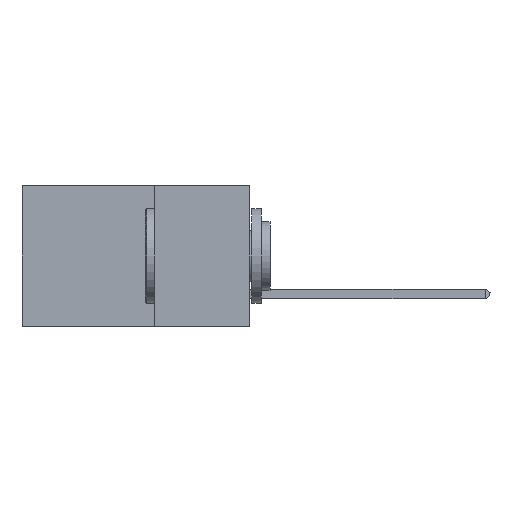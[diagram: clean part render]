
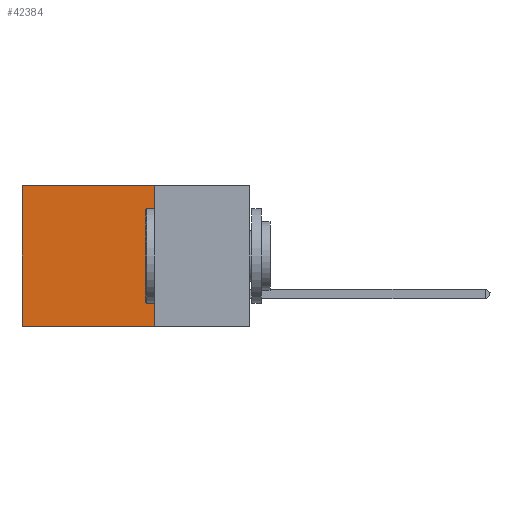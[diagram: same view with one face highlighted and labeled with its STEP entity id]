
A CAD part, left-side view. The second image highlights one B-rep face of the part: STEP entity #42384.
In plain terms, the highlighted planar face has unit normal (-1, 0, 0).
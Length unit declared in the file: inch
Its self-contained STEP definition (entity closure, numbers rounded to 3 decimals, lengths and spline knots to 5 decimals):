
#174 = EDGE_CURVE ( 'NONE', #48204, #36725, #38266, .T. ) ;
#1649 = PLANE ( 'NONE',  #5915 ) ;
#3595 = VERTEX_POINT ( 'NONE', #5203 ) ;
#3979 = VECTOR ( 'NONE', #16102, 39.37008 ) ;
#5203 = CARTESIAN_POINT ( 'NONE',  ( 0.2875, 0.25, -0.37 ) ) ;
#5599 = CARTESIAN_POINT ( 'NONE',  ( 0.2875, 0.25, 0. ) ) ;
#5915 = AXIS2_PLACEMENT_3D ( 'NONE', #5599, #47746, #28613 ) ;
#6799 = CARTESIAN_POINT ( 'NONE',  ( 0.2875, 0.25, -0.37 ) ) ;
#8748 = DIRECTION ( 'NONE',  ( 0., 1., 0. ) ) ;
#12864 = CARTESIAN_POINT ( 'NONE',  ( 0.2875, 0.6, 0. ) ) ;
#14858 = VERTEX_POINT ( 'NONE', #45023 ) ;
#14999 = ORIENTED_EDGE ( 'NONE', *, *, #17855, .F. ) ;
#16102 = DIRECTION ( 'NONE',  ( 0., 0., -1. ) ) ;
#17855 = EDGE_CURVE ( 'NONE', #48204, #3595, #39730, .T. ) ;
#18066 = VECTOR ( 'NONE', #48326, 39.37008 ) ;
#19684 = ORIENTED_EDGE ( 'NONE', *, *, #37822, .T. ) ;
#22387 = CARTESIAN_POINT ( 'NONE',  ( 0.2875, 0.6, 0. ) ) ;
#25393 = VECTOR ( 'NONE', #8748, 39.37008 ) ;
#27623 = CARTESIAN_POINT ( 'NONE',  ( 0.2875, 0.25, 0. ) ) ;
#28146 = ORIENTED_EDGE ( 'NONE', *, *, #39685, .F. ) ;
#28613 = DIRECTION ( 'NONE',  ( 0., 0., -1. ) ) ;
#32929 = FACE_OUTER_BOUND ( 'NONE', #34777, .T. ) ;
#34777 = EDGE_LOOP ( 'NONE', ( #19684, #28146, #14999, #37295 ) ) ;
#36725 = VERTEX_POINT ( 'NONE', #22387 ) ;
#37295 = ORIENTED_EDGE ( 'NONE', *, *, #174, .T. ) ;
#37822 = EDGE_CURVE ( 'NONE', #36725, #14858, #45231, .T. ) ;
#38220 = LINE ( 'NONE', #6799, #18066 ) ;
#38266 = LINE ( 'NONE', #40321, #25393 ) ;
#39685 = EDGE_CURVE ( 'NONE', #3595, #14858, #38220, .T. ) ;
#39730 = LINE ( 'NONE', #40845, #48812 ) ;
#40321 = CARTESIAN_POINT ( 'NONE',  ( 0.2875, 0.25, 0. ) ) ;
#40845 = CARTESIAN_POINT ( 'NONE',  ( 0.2875, 0.25, 0. ) ) ;
#42384 = ADVANCED_FACE ( 'NONE', ( #32929 ), #1649, .F. ) ;
#44358 = DIRECTION ( 'NONE',  ( 0., 0., -1. ) ) ;
#45023 = CARTESIAN_POINT ( 'NONE',  ( 0.2875, 0.6, -0.37 ) ) ;
#45231 = LINE ( 'NONE', #12864, #3979 ) ;
#47746 = DIRECTION ( 'NONE',  ( 1., 0., 0. ) ) ;
#48204 = VERTEX_POINT ( 'NONE', #27623 ) ;
#48326 = DIRECTION ( 'NONE',  ( 0., 1., 0. ) ) ;
#48812 = VECTOR ( 'NONE', #44358, 39.37008 ) ;
